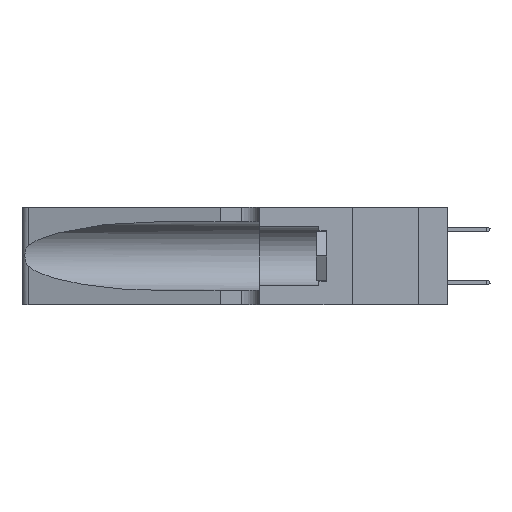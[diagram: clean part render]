
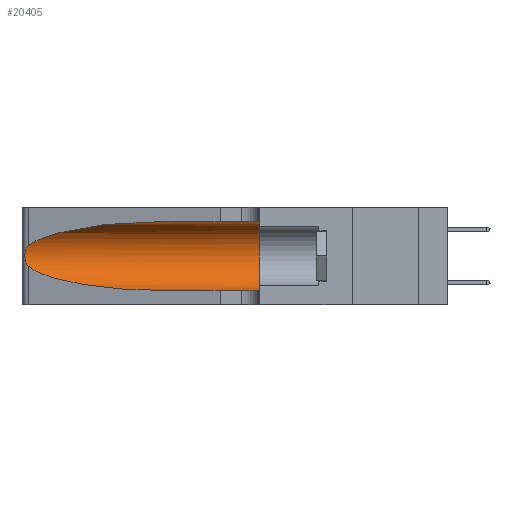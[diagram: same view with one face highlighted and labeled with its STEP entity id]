
A CAD part, left-side view. The second image highlights one B-rep face of the part: STEP entity #20405.
In plain terms, the highlighted cylindrical face has radius 3.308 mm (diameter 6.617 mm), a partial arc.
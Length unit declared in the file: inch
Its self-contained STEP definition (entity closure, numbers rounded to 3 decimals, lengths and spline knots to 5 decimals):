
#448 = EDGE_CURVE ( 'NONE', #29342, #3514, #5147, .T. ) ;
#904 = DIRECTION ( 'NONE',  ( 0., -1., 0. ) ) ;
#1123 = DIRECTION ( 'NONE',  ( 0., 0., 1. ) ) ;
#1399 = CARTESIAN_POINT ( 'NONE',  ( 0.1305, 1.61858, 0.31525 ) ) ;
#2569 =( BOUNDED_CURVE ( )  B_SPLINE_CURVE ( 3, ( #9767, #29180, #38386, #22688 ),
 .UNSPECIFIED., .F., .T. ) 
 B_SPLINE_CURVE_WITH_KNOTS ( ( 4, 4 ),
 ( 1.5708, 2.84003 ),
 .UNSPECIFIED. ) 
 CURVE ( )  GEOMETRIC_REPRESENTATION_ITEM ( )  RATIONAL_B_SPLINE_CURVE ( ( 1., 0.87, 0.87, 1. ) ) 
 REPRESENTATION_ITEM ( '' )  );
#3028 = VERTEX_POINT ( 'NONE', #6970 ) ;
#3514 = VERTEX_POINT ( 'NONE', #27831 ) ;
#4667 = ORIENTED_EDGE ( 'NONE', *, *, #17789, .F. ) ;
#5147 =( BOUNDED_CURVE ( )  B_SPLINE_CURVE ( 3, ( #22769, #32792, #36018, #36875 ),
 .UNSPECIFIED., .F., .F. ) 
 B_SPLINE_CURVE_WITH_KNOTS ( ( 4, 4 ),
 ( 3.44316, 4.71239 ),
 .UNSPECIFIED. ) 
 CURVE ( )  GEOMETRIC_REPRESENTATION_ITEM ( )  RATIONAL_B_SPLINE_CURVE ( ( 1., 0.87, 0.87, 1. ) ) 
 REPRESENTATION_ITEM ( '' )  );
#6390 = CARTESIAN_POINT ( 'NONE',  ( 0.25854, 1.2359, 0.20912 ) ) ;
#6970 = CARTESIAN_POINT ( 'NONE',  ( 0.1305, 0.35, 0.31525 ) ) ;
#7073 = CARTESIAN_POINT ( 'NONE',  ( 0.26017, 1.23833, 0.17102 ) ) ;
#8706 = CARTESIAN_POINT ( 'NONE',  ( 0.1305, 0.35, 0.05475 ) ) ;
#9769 = CARTESIAN_POINT ( 'NONE',  ( 0.26018, 1.23835, 0.19895 ) ) ;
#9767 = CARTESIAN_POINT ( 'NONE',  ( 0.1305, 0.72297, 0.31525 ) ) ;
#10005 = ORIENTED_EDGE ( 'NONE', *, *, #16010, .T. ) ;
#10383 = FACE_OUTER_BOUND ( 'NONE', #37039, .T. ) ;
#10473 = EDGE_CURVE ( 'NONE', #36087, #29342, #13114, .T. ) ;
#10941 = CARTESIAN_POINT ( 'NONE',  ( 0.1305, 1.61858, 0.185 ) ) ;
#11003 = DIRECTION ( 'NONE',  ( 0., 1., 0. ) ) ;
#11303 = AXIS2_PLACEMENT_3D ( 'NONE', #26723, #11003, #1123 ) ;
#12064 = EDGE_CURVE ( 'NONE', #3514, #34447, #14284, .T. ) ;
#13114 = B_SPLINE_CURVE_WITH_KNOTS ( 'NONE', 3,
 ( #13141, #32733, #25957, #16263, #6390, #9769, #26948, #39345, #7073, #33302, #39791, #39503, #35797, #29553 ),
 .UNSPECIFIED., .F., .F.,
 ( 4, 2, 2, 2, 2, 2, 4 ),
 ( 0., 0.00027, 0.00053, 0.00107, 0.0016, 0.00187, 0.00214 ),
 .UNSPECIFIED. ) ;
#13141 = CARTESIAN_POINT ( 'NONE',  ( 0.25487, 1.22718, 0.22369 ) ) ;
#14284 = LINE ( 'NONE', #26931, #23968 ) ;
#16010 = EDGE_CURVE ( 'NONE', #17814, #36087, #2569, .T. ) ;
#16263 = CARTESIAN_POINT ( 'NONE',  ( 0.25787, 1.23484, 0.2124 ) ) ;
#16403 = ORIENTED_EDGE ( 'NONE', *, *, #30276, .F. ) ;
#17789 = EDGE_CURVE ( 'NONE', #3028, #34447, #33446, .T. ) ;
#17814 = VERTEX_POINT ( 'NONE', #23471 ) ;
#17925 = LINE ( 'NONE', #1399, #38189 ) ;
#18978 = CYLINDRICAL_SURFACE ( 'NONE', #29727, 0.13025 ) ;
#20405 = ADVANCED_FACE ( 'NONE', ( #10383 ), #18978, .F. ) ;
#22688 = CARTESIAN_POINT ( 'NONE',  ( 0.25487, 1.22718, 0.22369 ) ) ;
#22769 = CARTESIAN_POINT ( 'NONE',  ( 0.25487, 1.22718, 0.14631 ) ) ;
#23471 = CARTESIAN_POINT ( 'NONE',  ( 0.1305, 0.72297, 0.31525 ) ) ;
#23968 = VECTOR ( 'NONE', #31163, 39.37008 ) ;
#25957 = CARTESIAN_POINT ( 'NONE',  ( 0.25639, 1.23184, 0.21858 ) ) ;
#26723 = CARTESIAN_POINT ( 'NONE',  ( 0.1305, 0.35, 0.185 ) ) ;
#26839 = ORIENTED_EDGE ( 'NONE', *, *, #12064, .T. ) ;
#26931 = CARTESIAN_POINT ( 'NONE',  ( 0.1305, 1.61858, 0.05475 ) ) ;
#26948 = CARTESIAN_POINT ( 'NONE',  ( 0.26075, 1.23896, 0.19203 ) ) ;
#27831 = CARTESIAN_POINT ( 'NONE',  ( 0.1305, 0.72297, 0.05475 ) ) ;
#29180 = CARTESIAN_POINT ( 'NONE',  ( 0.18966, 0.96281, 0.31525 ) ) ;
#29258 = ORIENTED_EDGE ( 'NONE', *, *, #448, .T. ) ;
#29342 = VERTEX_POINT ( 'NONE', #32373 ) ;
#29553 = CARTESIAN_POINT ( 'NONE',  ( 0.25487, 1.22718, 0.14631 ) ) ;
#29727 = AXIS2_PLACEMENT_3D ( 'NONE', #10941, #904, #33615 ) ;
#30276 = EDGE_CURVE ( 'NONE', #17814, #3028, #17925, .T. ) ;
#31163 = DIRECTION ( 'NONE',  ( 0., -1., 0. ) ) ;
#32373 = CARTESIAN_POINT ( 'NONE',  ( 0.25487, 1.22718, 0.14631 ) ) ;
#32733 = CARTESIAN_POINT ( 'NONE',  ( 0.25555, 1.22994, 0.2215 ) ) ;
#32792 = CARTESIAN_POINT ( 'NONE',  ( 0.2373, 1.15595, 0.08982 ) ) ;
#33302 = CARTESIAN_POINT ( 'NONE',  ( 0.25856, 1.23593, 0.16098 ) ) ;
#33446 = CIRCLE ( 'NONE', #11303, 0.13025 ) ;
#33615 = DIRECTION ( 'NONE',  ( 0., 0., -1. ) ) ;
#34447 = VERTEX_POINT ( 'NONE', #8706 ) ;
#34598 = ORIENTED_EDGE ( 'NONE', *, *, #10473, .T. ) ;
#35797 = CARTESIAN_POINT ( 'NONE',  ( 0.25555, 1.22993, 0.14849 ) ) ;
#36018 = CARTESIAN_POINT ( 'NONE',  ( 0.18966, 0.96281, 0.05475 ) ) ;
#36087 = VERTEX_POINT ( 'NONE', #38908 ) ;
#36875 = CARTESIAN_POINT ( 'NONE',  ( 0.1305, 0.72297, 0.05475 ) ) ;
#37028 = DIRECTION ( 'NONE',  ( 0., -1., 0. ) ) ;
#37039 = EDGE_LOOP ( 'NONE', ( #10005, #34598, #29258, #26839, #4667, #16403 ) ) ;
#38189 = VECTOR ( 'NONE', #37028, 39.37008 ) ;
#38386 = CARTESIAN_POINT ( 'NONE',  ( 0.2373, 1.15595, 0.28018 ) ) ;
#38908 = CARTESIAN_POINT ( 'NONE',  ( 0.25487, 1.22718, 0.22369 ) ) ;
#39345 = CARTESIAN_POINT ( 'NONE',  ( 0.26075, 1.23896, 0.178 ) ) ;
#39503 = CARTESIAN_POINT ( 'NONE',  ( 0.25639, 1.23186, 0.15144 ) ) ;
#39791 = CARTESIAN_POINT ( 'NONE',  ( 0.25789, 1.23486, 0.15765 ) ) ;
